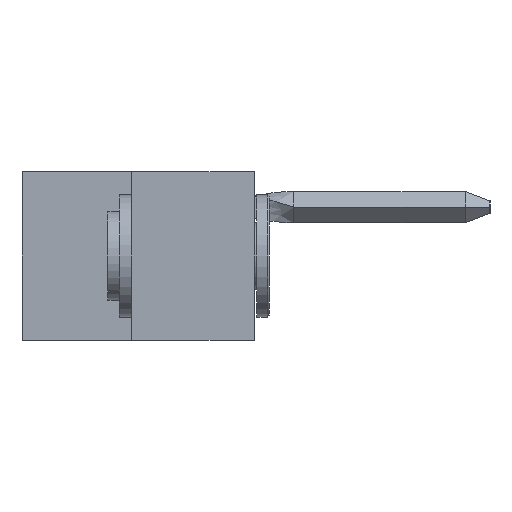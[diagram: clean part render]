
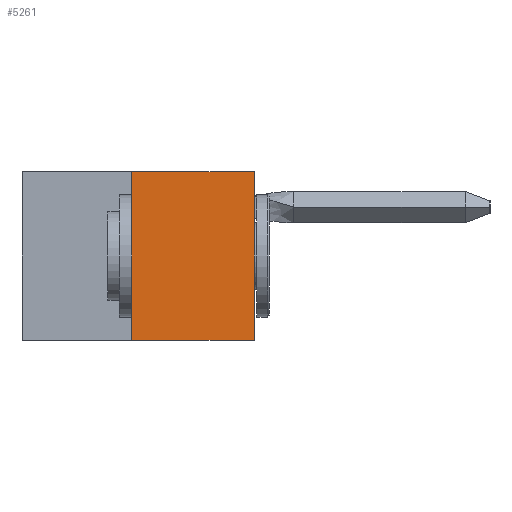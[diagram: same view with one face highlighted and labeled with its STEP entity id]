
A CAD part, left-side view. The second image highlights one B-rep face of the part: STEP entity #5261.
In plain terms, the highlighted planar face has unit normal (-1, 0, 0).
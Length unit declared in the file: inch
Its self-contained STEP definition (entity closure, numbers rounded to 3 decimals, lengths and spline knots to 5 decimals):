
#221 = ORIENTED_EDGE ( 'NONE', *, *, #37469, .T. ) ;
#735 = DIRECTION ( 'NONE',  ( 0., 0., 1. ) ) ;
#1618 = PLANE ( 'NONE',  #20954 ) ;
#2647 = CARTESIAN_POINT ( 'NONE',  ( 0., 0., 0. ) ) ;
#2927 = CARTESIAN_POINT ( 'NONE',  ( 0., 0.473, 0. ) ) ;
#2994 = VERTEX_POINT ( 'NONE', #3654 ) ;
#3053 = EDGE_LOOP ( 'NONE', ( #34939, #11020, #33216, #221 ) ) ;
#3654 = CARTESIAN_POINT ( 'NONE',  ( 0., 0.25, -0.343 ) ) ;
#5261 = ADVANCED_FACE ( 'NONE', ( #14695 ), #1618, .F. ) ;
#5963 = CARTESIAN_POINT ( 'NONE',  ( 0., 0.473, -0.343 ) ) ;
#7545 = DIRECTION ( 'NONE',  ( 1., 0., 0. ) ) ;
#8342 = LINE ( 'NONE', #2927, #24488 ) ;
#9055 = LINE ( 'NONE', #27272, #31591 ) ;
#11020 = ORIENTED_EDGE ( 'NONE', *, *, #22219, .F. ) ;
#13781 = CARTESIAN_POINT ( 'NONE',  ( 0., 0., 0. ) ) ;
#14695 = FACE_OUTER_BOUND ( 'NONE', #3053, .T. ) ;
#14814 = VERTEX_POINT ( 'NONE', #22227 ) ;
#15047 = VECTOR ( 'NONE', #35299, 39.37008 ) ;
#15985 = VERTEX_POINT ( 'NONE', #22912 ) ;
#17761 = VERTEX_POINT ( 'NONE', #13781 ) ;
#20954 = AXIS2_PLACEMENT_3D ( 'NONE', #33759, #7545, #31076 ) ;
#22219 = EDGE_CURVE ( 'NONE', #2994, #15985, #9055, .T. ) ;
#22227 = CARTESIAN_POINT ( 'NONE',  ( 0., 0., -0.343 ) ) ;
#22912 = CARTESIAN_POINT ( 'NONE',  ( 0., 0.25, 0. ) ) ;
#24488 = VECTOR ( 'NONE', #35206, 39.37008 ) ;
#27272 = CARTESIAN_POINT ( 'NONE',  ( 0., 0.25, 0. ) ) ;
#27877 = LINE ( 'NONE', #5963, #35175 ) ;
#29290 = LINE ( 'NONE', #2647, #15047 ) ;
#29644 = DIRECTION ( 'NONE',  ( 0., -1., 0. ) ) ;
#31076 = DIRECTION ( 'NONE',  ( 0., 0., -1. ) ) ;
#31591 = VECTOR ( 'NONE', #735, 39.37008 ) ;
#32679 = EDGE_CURVE ( 'NONE', #2994, #14814, #27877, .T. ) ;
#33216 = ORIENTED_EDGE ( 'NONE', *, *, #32679, .T. ) ;
#33759 = CARTESIAN_POINT ( 'NONE',  ( 0., 0.473, 0. ) ) ;
#34808 = EDGE_CURVE ( 'NONE', #15985, #17761, #8342, .T. ) ;
#34939 = ORIENTED_EDGE ( 'NONE', *, *, #34808, .F. ) ;
#35175 = VECTOR ( 'NONE', #29644, 39.37008 ) ;
#35206 = DIRECTION ( 'NONE',  ( 0., -1., 0. ) ) ;
#35299 = DIRECTION ( 'NONE',  ( 0., 0., 1. ) ) ;
#37469 = EDGE_CURVE ( 'NONE', #14814, #17761, #29290, .T. ) ;
